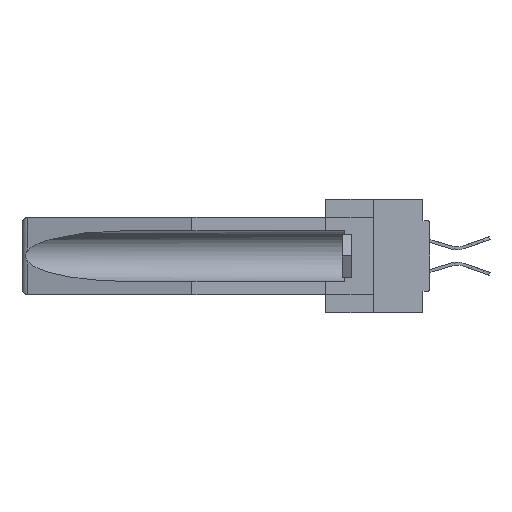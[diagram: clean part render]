
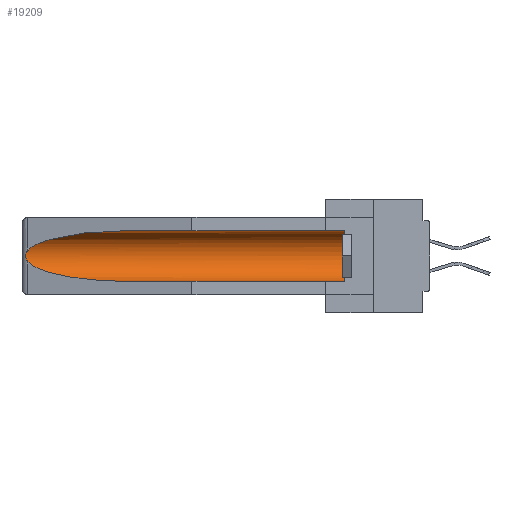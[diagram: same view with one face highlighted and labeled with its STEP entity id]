
A CAD part, left-side view. The second image highlights one B-rep face of the part: STEP entity #19209.
In plain terms, the highlighted cylindrical face has radius 2.857 mm (diameter 5.715 mm), a partial arc.
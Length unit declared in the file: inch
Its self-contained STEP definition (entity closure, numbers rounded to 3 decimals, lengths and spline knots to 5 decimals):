
#640 = CARTESIAN_POINT ( 'NONE',  ( 0.155, 0.126, -0.1715 ) ) ;
#2163 = CARTESIAN_POINT ( 'NONE',  ( 0.2675, 1.53308, -0.17534 ) ) ;
#2448 = VERTEX_POINT ( 'NONE', #3425 ) ;
#2561 = VERTEX_POINT ( 'NONE', #11024 ) ;
#2657 = DIRECTION ( 'NONE',  ( 0., 1., 0. ) ) ;
#3302 = CARTESIAN_POINT ( 'NONE',  ( 0.155, 0.126, -0.284 ) ) ;
#3425 = CARTESIAN_POINT ( 'NONE',  ( 0.155, 1.07973, -0.059 ) ) ;
#4040 = DIRECTION ( 'NONE',  ( 0., 1., 0. ) ) ;
#4256 = ORIENTED_EDGE ( 'NONE', *, *, #15129, .T. ) ;
#5058 = CARTESIAN_POINT ( 'NONE',  ( 0.26537, 1.52718, -0.19328 ) ) ;
#5100 = ORIENTED_EDGE ( 'NONE', *, *, #22013, .F. ) ;
#5280 = AXIS2_PLACEMENT_3D ( 'NONE', #23638, #4040, #32146 ) ;
#5882 = FACE_OUTER_BOUND ( 'NONE', #11863, .T. ) ;
#6241 = CARTESIAN_POINT ( 'NONE',  ( 0.21114, 1.30732, -0.059 ) ) ;
#7608 = CARTESIAN_POINT ( 'NONE',  ( 0.2673, 1.5327, -0.16383 ) ) ;
#9753 = CARTESIAN_POINT ( 'NONE',  ( 0.25451, 1.48313, -0.24835 ) ) ;
#11024 = CARTESIAN_POINT ( 'NONE',  ( 0.155, 1.07973, -0.284 ) ) ;
#11863 = EDGE_LOOP ( 'NONE', ( #25073, #14847, #13998, #5100, #4256, #34514 ) ) ;
#13998 = ORIENTED_EDGE ( 'NONE', *, *, #17893, .T. ) ;
#14301 = CARTESIAN_POINT ( 'NONE',  ( 0.155, 1.07973, -0.059 ) ) ;
#14847 = ORIENTED_EDGE ( 'NONE', *, *, #27436, .T. ) ;
#15129 = EDGE_CURVE ( 'NONE', #33549, #29264, #34138, .T. ) ;
#15252 = CARTESIAN_POINT ( 'NONE',  ( 0.26537, 1.52718, -0.14972 ) ) ;
#15490 = CYLINDRICAL_SURFACE ( 'NONE', #5280, 0.1125 ) ;
#16046 = CARTESIAN_POINT ( 'NONE',  ( 0.26597, 1.52961, -0.15275 ) ) ;
#17632 =( BOUNDED_CURVE ( )  B_SPLINE_CURVE ( 3, ( #14301, #6241, #22820, #30965 ),
 .UNSPECIFIED., .F., .F. ) 
 B_SPLINE_CURVE_WITH_KNOTS ( ( 4, 4 ),
 ( 4.71239, 6.08839 ),
 .UNSPECIFIED. ) 
 CURVE ( )  GEOMETRIC_REPRESENTATION_ITEM ( )  RATIONAL_B_SPLINE_CURVE ( ( 1., 0.848, 0.848, 1. ) ) 
 REPRESENTATION_ITEM ( '' )  );
#17729 = VERTEX_POINT ( 'NONE', #15252 ) ;
#17893 = EDGE_CURVE ( 'NONE', #31805, #2561, #18739, .T. ) ;
#18291 = CARTESIAN_POINT ( 'NONE',  ( 0.155, 1.07973, -0.284 ) ) ;
#18739 =( BOUNDED_CURVE ( )  B_SPLINE_CURVE ( 3, ( #28986, #9753, #29222, #18291 ),
 .UNSPECIFIED., .F., .F. ) 
 B_SPLINE_CURVE_WITH_KNOTS ( ( 4, 4 ),
 ( 0.1948, 1.5708 ),
 .UNSPECIFIED. ) 
 CURVE ( )  GEOMETRIC_REPRESENTATION_ITEM ( )  RATIONAL_B_SPLINE_CURVE ( ( 1., 0.848, 0.848, 1. ) ) 
 REPRESENTATION_ITEM ( '' )  );
#18832 = CARTESIAN_POINT ( 'NONE',  ( 0.26654, 1.53092, -0.15636 ) ) ;
#19209 = ADVANCED_FACE ( 'NONE', ( #5882 ), #15490, .F. ) ;
#19659 = DIRECTION ( 'NONE',  ( 0., 1., 0. ) ) ;
#20103 = DIRECTION ( 'NONE',  ( 0., -1., 0. ) ) ;
#20369 = VECTOR ( 'NONE', #2657, 39.37008 ) ;
#21632 = CARTESIAN_POINT ( 'NONE',  ( 0.2673, 1.53269, -0.17917 ) ) ;
#21755 = CARTESIAN_POINT ( 'NONE',  ( 0.26597, 1.5296, -0.19026 ) ) ;
#21934 = VECTOR ( 'NONE', #19659, 39.37008 ) ;
#22013 = EDGE_CURVE ( 'NONE', #33549, #2561, #28878, .T. ) ;
#22525 = B_SPLINE_CURVE_WITH_KNOTS ( 'NONE', 3,
 ( #30383, #16046, #18832, #7608, #27211, #2163, #21632, #35646, #21755, #5058 ),
 .UNSPECIFIED., .F., .F.,
 ( 4, 2, 2, 2, 4 ),
 ( 0., 0.00029, 0.00058, 0.00087, 0.00117 ),
 .UNSPECIFIED. ) ;
#22820 = CARTESIAN_POINT ( 'NONE',  ( 0.25451, 1.48313, -0.09465 ) ) ;
#23638 = CARTESIAN_POINT ( 'NONE',  ( 0.155, -0.30754, -0.1715 ) ) ;
#24796 = AXIS2_PLACEMENT_3D ( 'NONE', #640, #20103, #28616 ) ;
#25073 = ORIENTED_EDGE ( 'NONE', *, *, #35110, .T. ) ;
#25130 = LINE ( 'NONE', #27345, #20369 ) ;
#26857 = CARTESIAN_POINT ( 'NONE',  ( 0.26537, 1.52718, -0.19328 ) ) ;
#27211 = CARTESIAN_POINT ( 'NONE',  ( 0.2675, 1.53308, -0.16763 ) ) ;
#27345 = CARTESIAN_POINT ( 'NONE',  ( 0.155, -0.30754, -0.059 ) ) ;
#27436 = EDGE_CURVE ( 'NONE', #17729, #31805, #22525, .T. ) ;
#28507 = CARTESIAN_POINT ( 'NONE',  ( 0.155, 0.126, -0.059 ) ) ;
#28616 = DIRECTION ( 'NONE',  ( 0., 0., 1. ) ) ;
#28878 = LINE ( 'NONE', #31072, #21934 ) ;
#28986 = CARTESIAN_POINT ( 'NONE',  ( 0.26537, 1.52718, -0.19328 ) ) ;
#29222 = CARTESIAN_POINT ( 'NONE',  ( 0.21114, 1.30732, -0.284 ) ) ;
#29264 = VERTEX_POINT ( 'NONE', #28507 ) ;
#30383 = CARTESIAN_POINT ( 'NONE',  ( 0.26537, 1.52718, -0.14972 ) ) ;
#30965 = CARTESIAN_POINT ( 'NONE',  ( 0.26537, 1.52718, -0.14972 ) ) ;
#31072 = CARTESIAN_POINT ( 'NONE',  ( 0.155, -0.30754, -0.284 ) ) ;
#31805 = VERTEX_POINT ( 'NONE', #26857 ) ;
#32146 = DIRECTION ( 'NONE',  ( 0., 0., 1. ) ) ;
#33549 = VERTEX_POINT ( 'NONE', #3302 ) ;
#34138 = CIRCLE ( 'NONE', #24796, 0.1125 ) ;
#34514 = ORIENTED_EDGE ( 'NONE', *, *, #35867, .T. ) ;
#35110 = EDGE_CURVE ( 'NONE', #2448, #17729, #17632, .T. ) ;
#35646 = CARTESIAN_POINT ( 'NONE',  ( 0.26655, 1.53094, -0.18657 ) ) ;
#35867 = EDGE_CURVE ( 'NONE', #29264, #2448, #25130, .T. ) ;
